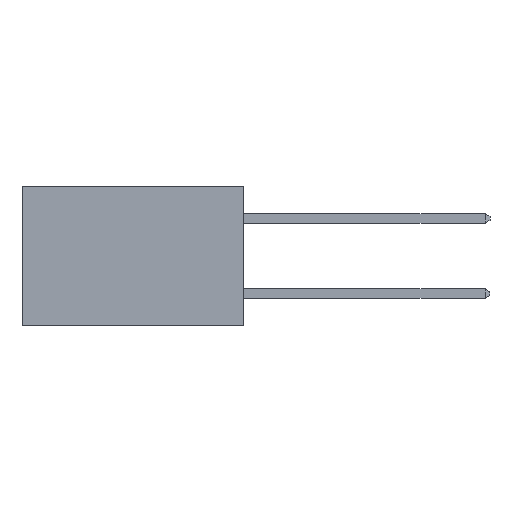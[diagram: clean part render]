
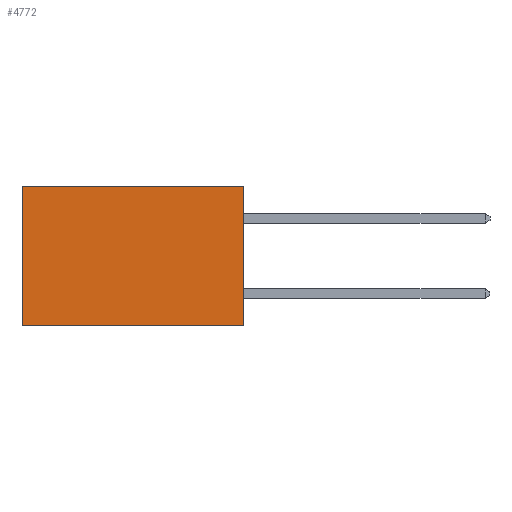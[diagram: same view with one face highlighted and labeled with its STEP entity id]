
A CAD part, left-side view. The second image highlights one B-rep face of the part: STEP entity #4772.
In plain terms, the highlighted planar face has unit normal (-1, 0, 0).
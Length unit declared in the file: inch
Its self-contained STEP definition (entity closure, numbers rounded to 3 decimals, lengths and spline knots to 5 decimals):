
#22 = VERTEX_POINT ( 'NONE', #13298 ) ;
#1160 = CARTESIAN_POINT ( 'NONE',  ( 0.277, 0.59, -0.37 ) ) ;
#1187 = EDGE_CURVE ( 'NONE', #6395, #2764, #9150, .T. ) ;
#1324 = VECTOR ( 'NONE', #8272, 39.37008 ) ;
#1363 = ORIENTED_EDGE ( 'NONE', *, *, #13447, .T. ) ;
#2024 = VERTEX_POINT ( 'NONE', #12251 ) ;
#2233 = DIRECTION ( 'NONE',  ( 0., 0., -1. ) ) ;
#2764 = VERTEX_POINT ( 'NONE', #11678 ) ;
#3017 = DIRECTION ( 'NONE',  ( 0., 1., 0. ) ) ;
#3049 = CARTESIAN_POINT ( 'NONE',  ( 0.277, 0., 0. ) ) ;
#3236 = CARTESIAN_POINT ( 'NONE',  ( 0.277, 0., -0.37 ) ) ;
#3247 = EDGE_CURVE ( 'NONE', #6395, #22, #6089, .T. ) ;
#3403 = VECTOR ( 'NONE', #5900, 39.37008 ) ;
#3845 = VECTOR ( 'NONE', #3017, 39.37008 ) ;
#4546 = LINE ( 'NONE', #8289, #1324 ) ;
#4771 = FACE_OUTER_BOUND ( 'NONE', #7837, .T. ) ;
#4772 = ADVANCED_FACE ( 'NONE', ( #4771 ), #9796, .F. ) ;
#5063 = LINE ( 'NONE', #1160, #10091 ) ;
#5900 = DIRECTION ( 'NONE',  ( 0., 0., -1. ) ) ;
#6089 = LINE ( 'NONE', #3049, #3845 ) ;
#6395 = VERTEX_POINT ( 'NONE', #8634 ) ;
#6425 = EDGE_CURVE ( 'NONE', #2764, #2024, #4546, .T. ) ;
#6643 = AXIS2_PLACEMENT_3D ( 'NONE', #10162, #9780, #9768 ) ;
#6797 = ORIENTED_EDGE ( 'NONE', *, *, #1187, .F. ) ;
#7837 = EDGE_LOOP ( 'NONE', ( #1363, #10295, #6797, #12640 ) ) ;
#8272 = DIRECTION ( 'NONE',  ( 0., 1., 0. ) ) ;
#8289 = CARTESIAN_POINT ( 'NONE',  ( 0.277, 0., -0.37 ) ) ;
#8634 = CARTESIAN_POINT ( 'NONE',  ( 0.277, 0., 0. ) ) ;
#9150 = LINE ( 'NONE', #3236, #3403 ) ;
#9768 = DIRECTION ( 'NONE',  ( 0., 0., -1. ) ) ;
#9780 = DIRECTION ( 'NONE',  ( 1., 0., 0. ) ) ;
#9796 = PLANE ( 'NONE',  #6643 ) ;
#10091 = VECTOR ( 'NONE', #2233, 39.37008 ) ;
#10162 = CARTESIAN_POINT ( 'NONE',  ( 0.277, 0., -0.37 ) ) ;
#10295 = ORIENTED_EDGE ( 'NONE', *, *, #6425, .F. ) ;
#11678 = CARTESIAN_POINT ( 'NONE',  ( 0.277, 0., -0.37 ) ) ;
#12251 = CARTESIAN_POINT ( 'NONE',  ( 0.277, 0.59, -0.37 ) ) ;
#12640 = ORIENTED_EDGE ( 'NONE', *, *, #3247, .T. ) ;
#13298 = CARTESIAN_POINT ( 'NONE',  ( 0.277, 0.59, 0. ) ) ;
#13447 = EDGE_CURVE ( 'NONE', #22, #2024, #5063, .T. ) ;
